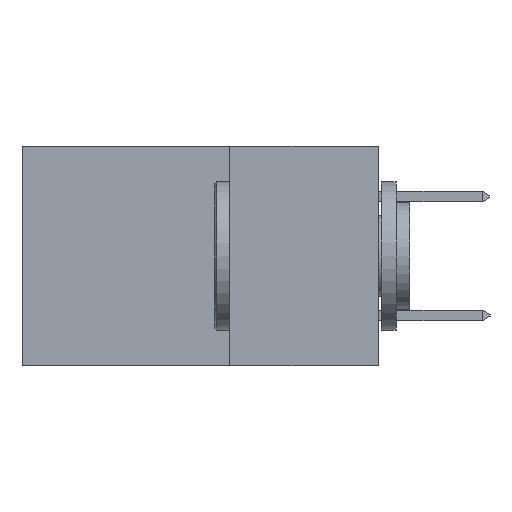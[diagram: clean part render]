
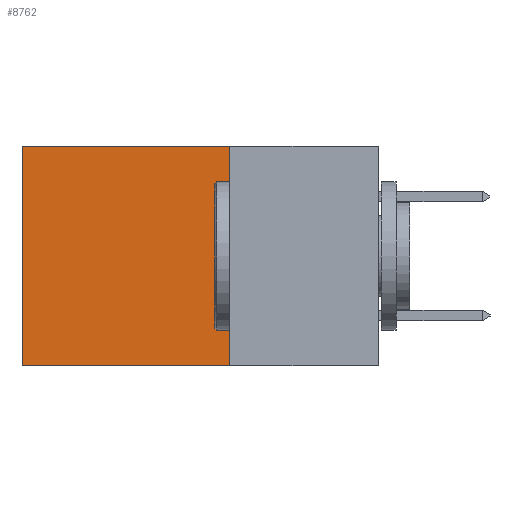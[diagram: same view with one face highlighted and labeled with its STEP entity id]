
A CAD part, left-side view. The second image highlights one B-rep face of the part: STEP entity #8762.
In plain terms, the highlighted planar face has unit normal (-1, 0, 0).
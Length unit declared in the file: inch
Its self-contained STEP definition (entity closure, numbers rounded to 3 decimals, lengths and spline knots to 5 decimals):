
#297 = DIRECTION ( 'NONE',  ( 1., 0., 0. ) ) ;
#304 = VECTOR ( 'NONE', #11941, 39.37008 ) ;
#1021 = CARTESIAN_POINT ( 'NONE',  ( 0.2615, 0.25, 0. ) ) ;
#1103 = CARTESIAN_POINT ( 'NONE',  ( 0.2615, 0.25, -0.37 ) ) ;
#1386 = DIRECTION ( 'NONE',  ( 0., 0., -1. ) ) ;
#1496 = DIRECTION ( 'NONE',  ( 0., 1., 0. ) ) ;
#2155 = VECTOR ( 'NONE', #1496, 39.37008 ) ;
#3177 = LINE ( 'NONE', #1103, #10846 ) ;
#3305 = LINE ( 'NONE', #4916, #304 ) ;
#3954 = EDGE_CURVE ( 'NONE', #9552, #11556, #9846, .T. ) ;
#4835 = CARTESIAN_POINT ( 'NONE',  ( 0.2615, 0.25, -0.37 ) ) ;
#4916 = CARTESIAN_POINT ( 'NONE',  ( 0.2615, 0.25, -0.37 ) ) ;
#5127 = EDGE_CURVE ( 'NONE', #11556, #12170, #6057, .T. ) ;
#5183 = ORIENTED_EDGE ( 'NONE', *, *, #5127, .T. ) ;
#5929 = AXIS2_PLACEMENT_3D ( 'NONE', #6336, #297, #7322 ) ;
#6057 = LINE ( 'NONE', #7375, #11034 ) ;
#6336 = CARTESIAN_POINT ( 'NONE',  ( 0.2615, 0.25, -0.37 ) ) ;
#6734 = ORIENTED_EDGE ( 'NONE', *, *, #3954, .T. ) ;
#7322 = DIRECTION ( 'NONE',  ( 0., 0., -1. ) ) ;
#7375 = CARTESIAN_POINT ( 'NONE',  ( 0.2615, 0.6, -0.37 ) ) ;
#7463 = CARTESIAN_POINT ( 'NONE',  ( 0.2615, 0.6, 0. ) ) ;
#8432 = CARTESIAN_POINT ( 'NONE',  ( 0.2615, 0.25, 0. ) ) ;
#8762 = ADVANCED_FACE ( 'NONE', ( #9135 ), #12269, .F. ) ;
#8974 = EDGE_LOOP ( 'NONE', ( #5183, #9632, #9684, #6734 ) ) ;
#9135 = FACE_OUTER_BOUND ( 'NONE', #8974, .T. ) ;
#9304 = EDGE_CURVE ( 'NONE', #9552, #9765, #3177, .T. ) ;
#9552 = VERTEX_POINT ( 'NONE', #8432 ) ;
#9632 = ORIENTED_EDGE ( 'NONE', *, *, #10577, .F. ) ;
#9684 = ORIENTED_EDGE ( 'NONE', *, *, #9304, .F. ) ;
#9765 = VERTEX_POINT ( 'NONE', #4835 ) ;
#9846 = LINE ( 'NONE', #1021, #2155 ) ;
#10155 = DIRECTION ( 'NONE',  ( 0., 0., -1. ) ) ;
#10577 = EDGE_CURVE ( 'NONE', #9765, #12170, #3305, .T. ) ;
#10846 = VECTOR ( 'NONE', #10155, 39.37008 ) ;
#11034 = VECTOR ( 'NONE', #1386, 39.37008 ) ;
#11556 = VERTEX_POINT ( 'NONE', #7463 ) ;
#11941 = DIRECTION ( 'NONE',  ( 0., 1., 0. ) ) ;
#12170 = VERTEX_POINT ( 'NONE', #12416 ) ;
#12269 = PLANE ( 'NONE',  #5929 ) ;
#12416 = CARTESIAN_POINT ( 'NONE',  ( 0.2615, 0.6, -0.37 ) ) ;
